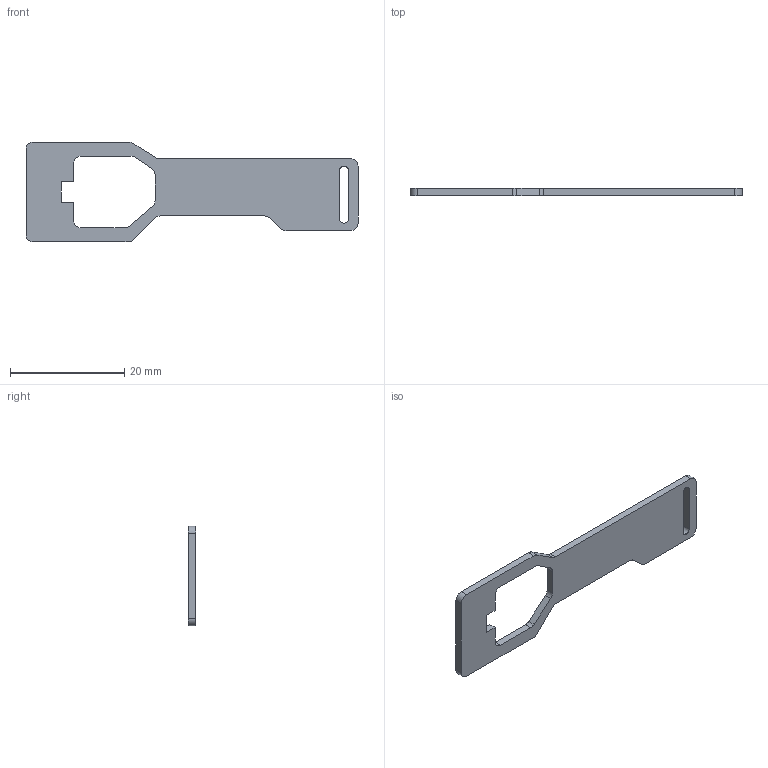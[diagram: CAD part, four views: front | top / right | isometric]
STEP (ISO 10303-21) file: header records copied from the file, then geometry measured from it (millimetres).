
FILE_DESCRIPTION (( 'STEP AP203' ), '1' );
FILE_NAME ('key.STEP', '2021-03-08T22:40:28', ( '' ), ( '' ), 'SwSTEP 2.0', 'SolidWorks 2019', '' );
FILE_SCHEMA (( 'CONFIG_CONTROL_DESIGN' ));
Length unit declared in the file: millimetre
Products named in the file (1): key
Bounding box: 58 x 1.3 x 17.45 mm (x, y, z)
Volume: 760.2 mm3; surface area: 1456.8 mm2
Topology: 1 solids, 1 shells, 43 faces, 123 edges, 82 vertices
Faces by surface type: plane 24, cylinder 19
Entity records: 1500 total; most frequent: DIRECTION 249, CARTESIAN_POINT 249, ORIENTED_EDGE 246, EDGE_CURVE 123, VECTOR 85, LINE 85, AXIS2_PLACEMENT_3D 82, VERTEX_POINT 82
